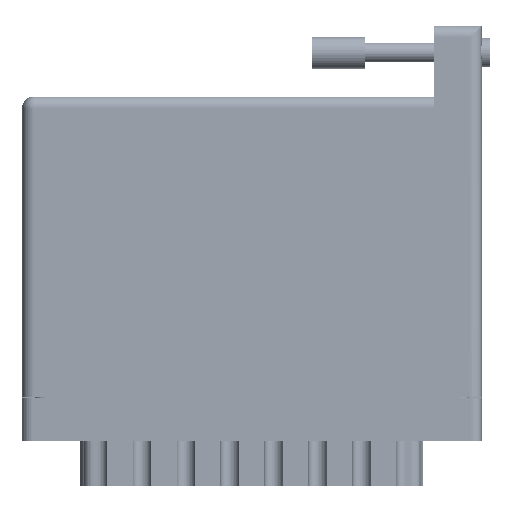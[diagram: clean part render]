
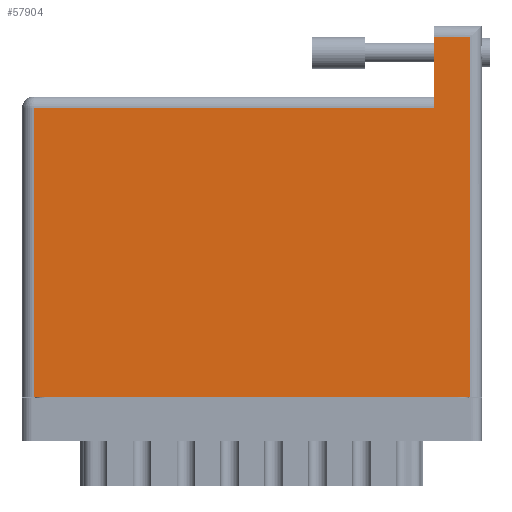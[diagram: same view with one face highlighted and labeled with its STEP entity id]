
A CAD part, front view. The second image highlights one B-rep face of the part: STEP entity #57904.
In plain terms, the highlighted face is planar.
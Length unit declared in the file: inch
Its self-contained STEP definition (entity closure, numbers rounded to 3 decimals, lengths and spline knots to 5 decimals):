
#84 = VECTOR ( 'NONE', #40750, 39.37008 ) ;
#666 = DIRECTION ( 'NONE',  ( 0., -1., 0. ) ) ;
#2088 = CARTESIAN_POINT ( 'NONE',  ( 0., 2.125, 0. ) ) ;
#4013 = LINE ( 'NONE', #2088, #32112 ) ;
#5545 = CARTESIAN_POINT ( 'NONE',  ( 0.07, 0., 0. ) ) ;
#7216 = CARTESIAN_POINT ( 'NONE',  ( 2.648, 0., 0. ) ) ;
#7566 = ORIENTED_EDGE ( 'NONE', *, *, #7686, .T. ) ;
#7686 = EDGE_CURVE ( 'NONE', #57991, #61092, #40341, .T. ) ;
#7727 = DIRECTION ( 'NONE',  ( -1., 0., 0. ) ) ;
#11397 = ORIENTED_EDGE ( 'NONE', *, *, #25784, .T. ) ;
#12146 = EDGE_CURVE ( 'NONE', #61092, #39470, #55678, .T. ) ;
#13523 = CARTESIAN_POINT ( 'NONE',  ( 0., 1.775, 0. ) ) ;
#14135 = EDGE_CURVE ( 'NONE', #42541, #62301, #34299, .T. ) ;
#14914 = ORIENTED_EDGE ( 'NONE', *, *, #12146, .T. ) ;
#18550 = CARTESIAN_POINT ( 'NONE',  ( 2.648, 2.195, 0. ) ) ;
#24675 = ORIENTED_EDGE ( 'NONE', *, *, #57295, .T. ) ;
#25420 = VECTOR ( 'NONE', #666, 39.37008 ) ;
#25560 = DIRECTION ( 'NONE',  ( 0., 0., -1. ) ) ;
#25784 = EDGE_CURVE ( 'NONE', #62301, #57991, #48544, .T. ) ;
#28481 = VECTOR ( 'NONE', #65668, 39.37008 ) ;
#28669 = CARTESIAN_POINT ( 'NONE',  ( 0.07, 0., 0. ) ) ;
#29952 = CARTESIAN_POINT ( 'NONE',  ( 2.438, 2.195, 0. ) ) ;
#32112 = VECTOR ( 'NONE', #7727, 39.37008 ) ;
#32710 = CARTESIAN_POINT ( 'NONE',  ( 2.648, 2.125, 0. ) ) ;
#33604 = VECTOR ( 'NONE', #56888, 39.37008 ) ;
#34299 = LINE ( 'NONE', #29952, #84 ) ;
#37092 = AXIS2_PLACEMENT_3D ( 'NONE', #13523, #25560, #64545 ) ;
#37458 = CARTESIAN_POINT ( 'NONE',  ( 0., 0., 0. ) ) ;
#39470 = VERTEX_POINT ( 'NONE', #7216 ) ;
#40341 = LINE ( 'NONE', #28669, #25420 ) ;
#40750 = DIRECTION ( 'NONE',  ( 0., -1., 0. ) ) ;
#42541 = VERTEX_POINT ( 'NONE', #48935 ) ;
#43673 = EDGE_LOOP ( 'NONE', ( #11397, #7566, #14914, #59675, #24675, #61593 ) ) ;
#46338 = CARTESIAN_POINT ( 'NONE',  ( 0., 1.705, 0. ) ) ;
#47133 = PLANE ( 'NONE',  #37092 ) ;
#47868 = CARTESIAN_POINT ( 'NONE',  ( 0.07, 1.705, 0. ) ) ;
#48544 = LINE ( 'NONE', #46338, #33604 ) ;
#48935 = CARTESIAN_POINT ( 'NONE',  ( 2.438, 2.125, 0. ) ) ;
#48942 = LINE ( 'NONE', #18550, #64703 ) ;
#55678 = LINE ( 'NONE', #37458, #28481 ) ;
#56888 = DIRECTION ( 'NONE',  ( -1., 0., 0. ) ) ;
#57295 = EDGE_CURVE ( 'NONE', #57565, #42541, #4013, .T. ) ;
#57565 = VERTEX_POINT ( 'NONE', #32710 ) ;
#57904 = ADVANCED_FACE ( 'NONE', ( #71519 ), #47133, .F. ) ;
#57991 = VERTEX_POINT ( 'NONE', #47868 ) ;
#59675 = ORIENTED_EDGE ( 'NONE', *, *, #72345, .T. ) ;
#61092 = VERTEX_POINT ( 'NONE', #5545 ) ;
#61593 = ORIENTED_EDGE ( 'NONE', *, *, #14135, .T. ) ;
#62301 = VERTEX_POINT ( 'NONE', #65891 ) ;
#62459 = DIRECTION ( 'NONE',  ( 0., 1., 0. ) ) ;
#64545 = DIRECTION ( 'NONE',  ( -1., 0., 0. ) ) ;
#64703 = VECTOR ( 'NONE', #62459, 39.37008 ) ;
#65668 = DIRECTION ( 'NONE',  ( 1., 0., 0. ) ) ;
#65891 = CARTESIAN_POINT ( 'NONE',  ( 2.438, 1.705, 0. ) ) ;
#71519 = FACE_OUTER_BOUND ( 'NONE', #43673, .T. ) ;
#72345 = EDGE_CURVE ( 'NONE', #39470, #57565, #48942, .T. ) ;
